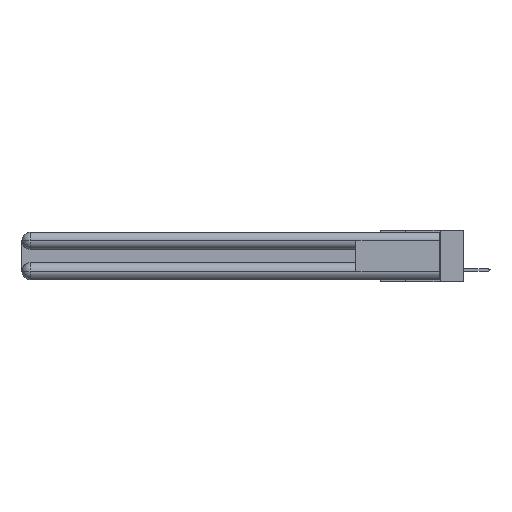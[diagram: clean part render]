
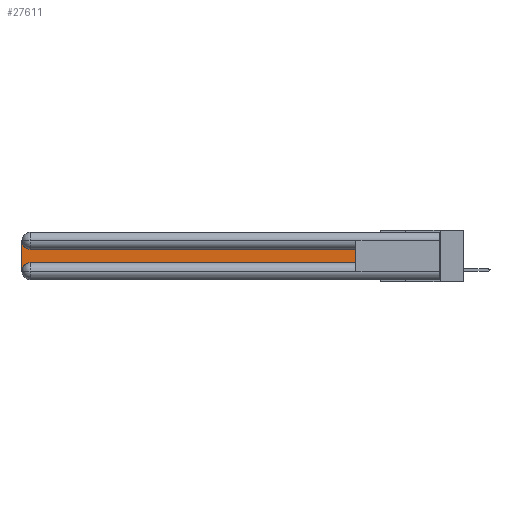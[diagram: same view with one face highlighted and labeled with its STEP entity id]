
A CAD part, left-side view. The second image highlights one B-rep face of the part: STEP entity #27611.
In plain terms, the highlighted planar face has unit normal (-1, 0, 0).
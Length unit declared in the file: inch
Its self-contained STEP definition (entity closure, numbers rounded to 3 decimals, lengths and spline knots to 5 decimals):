
#692 = EDGE_CURVE ( 'NONE', #30496, #9443, #19821, .T. ) ;
#1167 = EDGE_LOOP ( 'NONE', ( #11738, #13440, #31888, #16509, #6950, #17274 ) ) ;
#1339 = VECTOR ( 'NONE', #26360, 39.37008 ) ;
#1523 = LINE ( 'NONE', #31711, #21030 ) ;
#2316 = DIRECTION ( 'NONE',  ( 1., 0., 0. ) ) ;
#2361 = EDGE_CURVE ( 'NONE', #9443, #14220, #31283, .T. ) ;
#4152 = FACE_OUTER_BOUND ( 'NONE', #1167, .T. ) ;
#4166 = EDGE_CURVE ( 'NONE', #10718, #20383, #7348, .T. ) ;
#5093 = EDGE_CURVE ( 'NONE', #14220, #10718, #14408, .T. ) ;
#5595 = DIRECTION ( 'NONE',  ( 1., 0., 0. ) ) ;
#5764 = CARTESIAN_POINT ( 'NONE',  ( 0.075, 2.94, -0.0625 ) ) ;
#6200 = CARTESIAN_POINT ( 'NONE',  ( 0.075, 0.6, -0.1225 ) ) ;
#6950 = ORIENTED_EDGE ( 'NONE', *, *, #4166, .T. ) ;
#7317 = AXIS2_PLACEMENT_3D ( 'NONE', #30976, #5595, #10808 ) ;
#7348 = LINE ( 'NONE', #23919, #1339 ) ;
#8691 = DIRECTION ( 'NONE',  ( 0., 0., 1. ) ) ;
#9443 = VERTEX_POINT ( 'NONE', #31366 ) ;
#9476 = EDGE_CURVE ( 'NONE', #23911, #30496, #28313, .T. ) ;
#9943 = AXIS2_PLACEMENT_3D ( 'NONE', #5764, #28810, #31273 ) ;
#10718 = VERTEX_POINT ( 'NONE', #26063 ) ;
#10808 = DIRECTION ( 'NONE',  ( 0., 0., -1. ) ) ;
#11738 = ORIENTED_EDGE ( 'NONE', *, *, #9476, .T. ) ;
#13055 = PLANE ( 'NONE',  #7317 ) ;
#13440 = ORIENTED_EDGE ( 'NONE', *, *, #692, .T. ) ;
#14220 = VERTEX_POINT ( 'NONE', #32905 ) ;
#14408 = CIRCLE ( 'NONE', #17707, 0.06 ) ;
#14704 = CARTESIAN_POINT ( 'NONE',  ( 0.075, 2.94, -0.2775 ) ) ;
#16509 = ORIENTED_EDGE ( 'NONE', *, *, #5093, .T. ) ;
#17243 = CARTESIAN_POINT ( 'NONE',  ( 0.075, 0.6, -0.1225 ) ) ;
#17274 = ORIENTED_EDGE ( 'NONE', *, *, #18856, .T. ) ;
#17707 = AXIS2_PLACEMENT_3D ( 'NONE', #14704, #2316, #32757 ) ;
#18856 = EDGE_CURVE ( 'NONE', #20383, #23911, #1523, .T. ) ;
#19821 = CIRCLE ( 'NONE', #9943, 0.06 ) ;
#20383 = VERTEX_POINT ( 'NONE', #22888 ) ;
#21030 = VECTOR ( 'NONE', #8691, 39.37008 ) ;
#22888 = CARTESIAN_POINT ( 'NONE',  ( 0.075, 0.6, -0.2175 ) ) ;
#23911 = VERTEX_POINT ( 'NONE', #17243 ) ;
#23919 = CARTESIAN_POINT ( 'NONE',  ( 0.075, 0.6, -0.2175 ) ) ;
#24745 = VECTOR ( 'NONE', #31263, 39.37008 ) ;
#25017 = CARTESIAN_POINT ( 'NONE',  ( 0.075, 3., -0.2175 ) ) ;
#26063 = CARTESIAN_POINT ( 'NONE',  ( 0.075, 2.94, -0.2175 ) ) ;
#26360 = DIRECTION ( 'NONE',  ( 0., -1., 0. ) ) ;
#26866 = CARTESIAN_POINT ( 'NONE',  ( 0.075, 2.94, -0.1225 ) ) ;
#27611 = ADVANCED_FACE ( 'NONE', ( #4152 ), #13055, .F. ) ;
#28006 = DIRECTION ( 'NONE',  ( 0., 0., -1. ) ) ;
#28313 = LINE ( 'NONE', #6200, #24745 ) ;
#28810 = DIRECTION ( 'NONE',  ( 1., 0., 0. ) ) ;
#30496 = VERTEX_POINT ( 'NONE', #26866 ) ;
#30976 = CARTESIAN_POINT ( 'NONE',  ( 0.075, 3., -0.1225 ) ) ;
#31263 = DIRECTION ( 'NONE',  ( 0., 1., 0. ) ) ;
#31273 = DIRECTION ( 'NONE',  ( 0., 0., -1. ) ) ;
#31283 = LINE ( 'NONE', #25017, #31647 ) ;
#31366 = CARTESIAN_POINT ( 'NONE',  ( 0.075, 3., -0.0625 ) ) ;
#31647 = VECTOR ( 'NONE', #28006, 39.37008 ) ;
#31711 = CARTESIAN_POINT ( 'NONE',  ( 0.075, 0.6, -0.2175 ) ) ;
#31888 = ORIENTED_EDGE ( 'NONE', *, *, #2361, .T. ) ;
#32757 = DIRECTION ( 'NONE',  ( 0., 0., -1. ) ) ;
#32905 = CARTESIAN_POINT ( 'NONE',  ( 0.075, 3., -0.2775 ) ) ;
